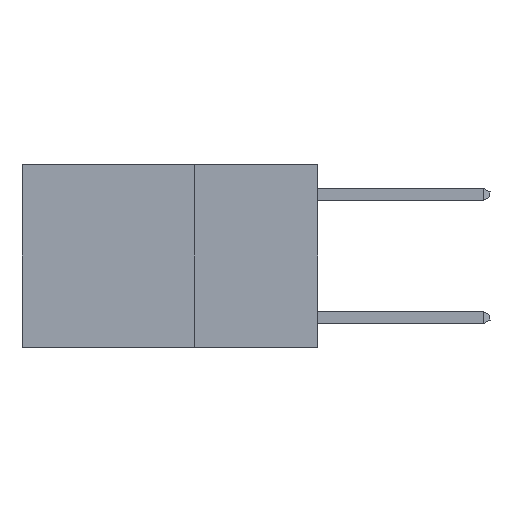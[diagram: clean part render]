
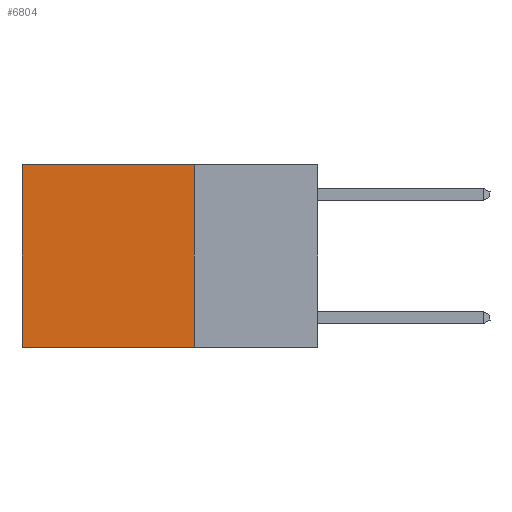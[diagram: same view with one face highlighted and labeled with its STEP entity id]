
A CAD part, left-side view. The second image highlights one B-rep face of the part: STEP entity #6804.
In plain terms, the highlighted planar face has unit normal (-1, 0, 0).
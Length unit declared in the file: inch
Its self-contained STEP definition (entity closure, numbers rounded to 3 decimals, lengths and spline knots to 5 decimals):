
#70 = EDGE_CURVE ( 'NONE', #14899, #17905, #20307, .T. ) ;
#83 = VERTEX_POINT ( 'NONE', #3167 ) ;
#215 = FACE_OUTER_BOUND ( 'NONE', #2264, .T. ) ;
#669 = VECTOR ( 'NONE', #24199, 39.37008 ) ;
#715 = LINE ( 'NONE', #6404, #16500 ) ;
#920 = ORIENTED_EDGE ( 'NONE', *, *, #2750, .T. ) ;
#2182 = CARTESIAN_POINT ( 'NONE',  ( 0.2625, 0.25, -0.37 ) ) ;
#2264 = EDGE_LOOP ( 'NONE', ( #920, #7460, #17041, #23881 ) ) ;
#2750 = EDGE_CURVE ( 'NONE', #17905, #83, #9098, .T. ) ;
#3167 = CARTESIAN_POINT ( 'NONE',  ( 0.2625, 0.6, -0.37 ) ) ;
#5040 = CARTESIAN_POINT ( 'NONE',  ( 0.2625, 0.6, 0. ) ) ;
#5442 = LINE ( 'NONE', #11075, #669 ) ;
#6038 = CARTESIAN_POINT ( 'NONE',  ( 0.2625, 0.25, 0. ) ) ;
#6232 = VERTEX_POINT ( 'NONE', #2182 ) ;
#6404 = CARTESIAN_POINT ( 'NONE',  ( 0.2625, 0.25, -0.37 ) ) ;
#6804 = ADVANCED_FACE ( 'NONE', ( #215 ), #7719, .F. ) ;
#7460 = ORIENTED_EDGE ( 'NONE', *, *, #21315, .F. ) ;
#7719 = PLANE ( 'NONE',  #18527 ) ;
#7993 = VECTOR ( 'NONE', #22064, 39.37008 ) ;
#9098 = LINE ( 'NONE', #5040, #24172 ) ;
#11075 = CARTESIAN_POINT ( 'NONE',  ( 0.2625, 0.25, 0. ) ) ;
#11828 = EDGE_CURVE ( 'NONE', #14899, #6232, #5442, .T. ) ;
#14899 = VERTEX_POINT ( 'NONE', #6038 ) ;
#15184 = CARTESIAN_POINT ( 'NONE',  ( 0.2625, 0.25, 0. ) ) ;
#16500 = VECTOR ( 'NONE', #19475, 39.37008 ) ;
#17041 = ORIENTED_EDGE ( 'NONE', *, *, #11828, .F. ) ;
#17754 = DIRECTION ( 'NONE',  ( 0., 0., -1. ) ) ;
#17905 = VERTEX_POINT ( 'NONE', #22555 ) ;
#18527 = AXIS2_PLACEMENT_3D ( 'NONE', #15184, #22664, #17754 ) ;
#19475 = DIRECTION ( 'NONE',  ( 0., 1., 0. ) ) ;
#20216 = DIRECTION ( 'NONE',  ( 0., 0., -1. ) ) ;
#20307 = LINE ( 'NONE', #21817, #7993 ) ;
#21315 = EDGE_CURVE ( 'NONE', #6232, #83, #715, .T. ) ;
#21817 = CARTESIAN_POINT ( 'NONE',  ( 0.2625, 0.25, 0. ) ) ;
#22064 = DIRECTION ( 'NONE',  ( 0., 1., 0. ) ) ;
#22555 = CARTESIAN_POINT ( 'NONE',  ( 0.2625, 0.6, 0. ) ) ;
#22664 = DIRECTION ( 'NONE',  ( 1., 0., 0. ) ) ;
#23881 = ORIENTED_EDGE ( 'NONE', *, *, #70, .T. ) ;
#24172 = VECTOR ( 'NONE', #20216, 39.37008 ) ;
#24199 = DIRECTION ( 'NONE',  ( 0., 0., -1. ) ) ;
